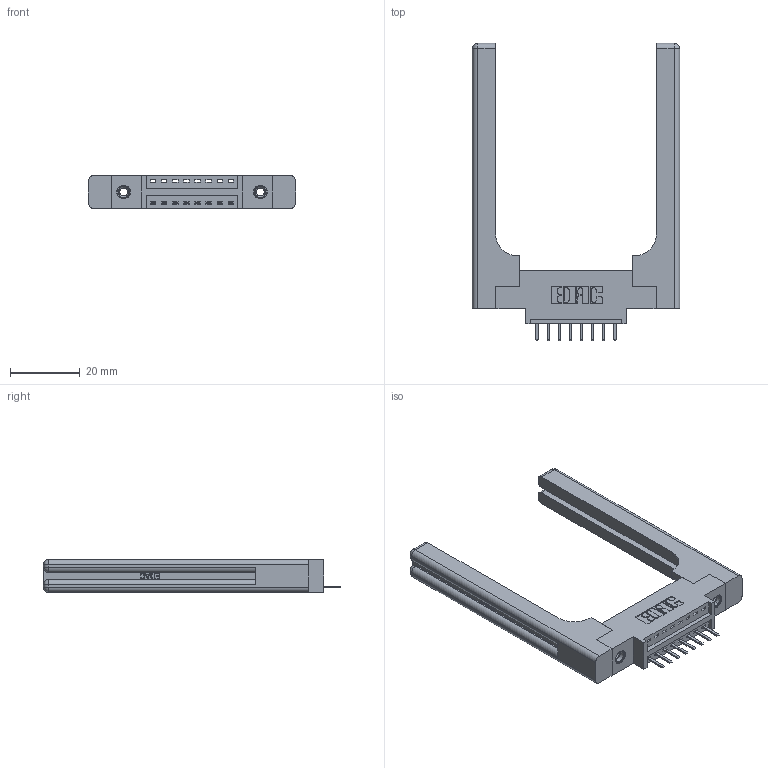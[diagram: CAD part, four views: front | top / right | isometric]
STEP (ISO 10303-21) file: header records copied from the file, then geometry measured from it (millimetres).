
FILE_DESCRIPTION (( 'STEP AP203' ), '1' );
FILE_NAME ('396-008-520-658.STEP', '2019-10-25T18:39:47', ( '' ), ( '' ), 'SwSTEP 2.0', 'SolidWorks 2016', '' );
FILE_SCHEMA (( 'CONFIG_CONTROL_DESIGN' ));
Length unit declared in the file: inch
Products named in the file (5): 346 Part_0.170 Offset - 0.156 Dia-TH; 346-220-058_345-220-058; 396-008-520-658; 345-292-001_345-293-120; 345-250-001_345-250-001-102
Assembly tree (13 placements, depth 2):
  396-008-520-658
    346 Part_0.170 Offset - 0.156 Dia-TH
    345-292-001_345-293-120  x8
    345-250-001_345-250-001-102  x2
    346-220-058_345-220-058  x2
Bounding box: 59.46 x 85.29 x 9.4 mm (x, y, z)
Volume: 12798.3 mm3; surface area: 11485.3 mm2
Topology: 13 solids, 13 shells, 878 faces, 2479 edges, 1610 vertices
Faces by surface type: plane 564, cylinder 254, bspline 36, cone 12, sphere 8, torus 4
Entity records: 14970 total; most frequent: CARTESIAN_POINT 3569, ORIENTED_EDGE 2296, DIRECTION 2108, EDGE_CURVE 1148, LINE 888, VECTOR 888, VERTEX_POINT 754, AXIS2_PLACEMENT_3D 610
